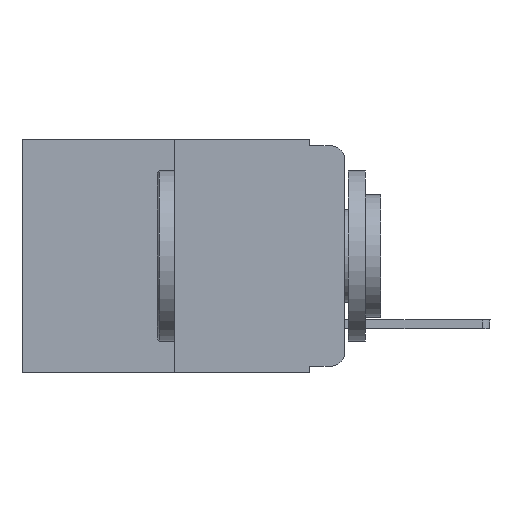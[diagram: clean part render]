
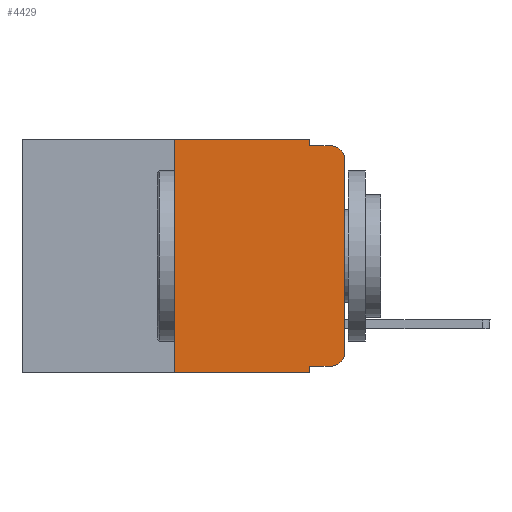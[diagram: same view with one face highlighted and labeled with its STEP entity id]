
A CAD part, left-side view. The second image highlights one B-rep face of the part: STEP entity #4429.
In plain terms, the highlighted planar face has unit normal (-1, 0, 0).
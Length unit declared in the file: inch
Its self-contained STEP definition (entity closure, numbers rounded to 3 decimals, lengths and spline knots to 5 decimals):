
#140 = VERTEX_POINT ( 'NONE', #6295 ) ;
#199 = ORIENTED_EDGE ( 'NONE', *, *, #9399, .T. ) ;
#248 = EDGE_CURVE ( 'NONE', #2056, #353, #7643, .T. ) ;
#317 = CIRCLE ( 'NONE', #6885, 0.02 ) ;
#353 = VERTEX_POINT ( 'NONE', #11382 ) ;
#426 = VECTOR ( 'NONE', #5553, 39.37008 ) ;
#587 = CARTESIAN_POINT ( 'NONE',  ( 0., 0.25, 0. ) ) ;
#712 = FACE_OUTER_BOUND ( 'NONE', #11468, .T. ) ;
#1334 = DIRECTION ( 'NONE',  ( 0., 0., -1. ) ) ;
#1338 = CARTESIAN_POINT ( 'NONE',  ( 0., 0.051, -0.01 ) ) ;
#1435 = CARTESIAN_POINT ( 'NONE',  ( 0., 0., 0. ) ) ;
#1440 = VERTEX_POINT ( 'NONE', #3270 ) ;
#1649 = CARTESIAN_POINT ( 'NONE',  ( 0., 0.02, -0.313 ) ) ;
#1845 = EDGE_CURVE ( 'NONE', #9660, #1440, #3730, .T. ) ;
#2056 = VERTEX_POINT ( 'NONE', #587 ) ;
#2116 = ORIENTED_EDGE ( 'NONE', *, *, #4659, .F. ) ;
#2437 = DIRECTION ( 'NONE',  ( 0., 0., 1. ) ) ;
#2562 = LINE ( 'NONE', #1435, #10126 ) ;
#3213 = EDGE_CURVE ( 'NONE', #9003, #10331, #8303, .T. ) ;
#3270 = CARTESIAN_POINT ( 'NONE',  ( 0., 0.02, -0.01 ) ) ;
#3324 = VECTOR ( 'NONE', #6934, 39.37008 ) ;
#3371 = DIRECTION ( 'NONE',  ( 0., -1., 0. ) ) ;
#3472 = VERTEX_POINT ( 'NONE', #9211 ) ;
#3614 = DIRECTION ( 'NONE',  ( 0., 0., -1. ) ) ;
#3730 = LINE ( 'NONE', #1338, #6246 ) ;
#3809 = CARTESIAN_POINT ( 'NONE',  ( 0., 0.02, -0.333 ) ) ;
#3892 = ORIENTED_EDGE ( 'NONE', *, *, #1845, .F. ) ;
#4140 = EDGE_CURVE ( 'NONE', #9003, #140, #12476, .T. ) ;
#4429 = ADVANCED_FACE ( 'NONE', ( #712 ), #6702, .F. ) ;
#4484 = VECTOR ( 'NONE', #7977, 39.37008 ) ;
#4570 = ORIENTED_EDGE ( 'NONE', *, *, #7966, .T. ) ;
#4659 = EDGE_CURVE ( 'NONE', #353, #9660, #10275, .T. ) ;
#4770 = DIRECTION ( 'NONE',  ( 1., 0., 0. ) ) ;
#4822 = DIRECTION ( 'NONE',  ( 0., 0., -1. ) ) ;
#5032 = VECTOR ( 'NONE', #3371, 39.37008 ) ;
#5109 = CARTESIAN_POINT ( 'NONE',  ( 0., 0.051, -0.333 ) ) ;
#5352 = VECTOR ( 'NONE', #7853, 39.37008 ) ;
#5553 = DIRECTION ( 'NONE',  ( 0., -1., 0. ) ) ;
#5767 = DIRECTION ( 'NONE',  ( 0., 0., -1. ) ) ;
#5954 = CARTESIAN_POINT ( 'NONE',  ( 0., 0.051, 0. ) ) ;
#6224 = CARTESIAN_POINT ( 'NONE',  ( 0., 0.25, -0.343 ) ) ;
#6246 = VECTOR ( 'NONE', #12232, 39.37008 ) ;
#6295 = CARTESIAN_POINT ( 'NONE',  ( 0., 0.051, -0.343 ) ) ;
#6491 = AXIS2_PLACEMENT_3D ( 'NONE', #11656, #4770, #4822 ) ;
#6660 = ORIENTED_EDGE ( 'NONE', *, *, #9619, .F. ) ;
#6702 = PLANE ( 'NONE',  #6491 ) ;
#6885 = AXIS2_PLACEMENT_3D ( 'NONE', #1649, #8663, #3614 ) ;
#6934 = DIRECTION ( 'NONE',  ( 0., 0., -1. ) ) ;
#6960 = VERTEX_POINT ( 'NONE', #6224 ) ;
#7109 = LINE ( 'NONE', #11032, #4484 ) ;
#7509 = VECTOR ( 'NONE', #1334, 39.37008 ) ;
#7643 = LINE ( 'NONE', #9274, #5032 ) ;
#7788 = CARTESIAN_POINT ( 'NONE',  ( 0., 0.051, -0.01 ) ) ;
#7853 = DIRECTION ( 'NONE',  ( 0., 0., 1. ) ) ;
#7945 = LINE ( 'NONE', #9692, #5352 ) ;
#7966 = EDGE_CURVE ( 'NONE', #10331, #10767, #317, .T. ) ;
#7977 = DIRECTION ( 'NONE',  ( 0., -1., 0. ) ) ;
#8023 = CARTESIAN_POINT ( 'NONE',  ( 0., 0.051, 0. ) ) ;
#8287 = ORIENTED_EDGE ( 'NONE', *, *, #3213, .T. ) ;
#8303 = LINE ( 'NONE', #11632, #426 ) ;
#8586 = AXIS2_PLACEMENT_3D ( 'NONE', #11627, #11546, #5767 ) ;
#8663 = DIRECTION ( 'NONE',  ( -1., 0., 0. ) ) ;
#8929 = EDGE_CURVE ( 'NONE', #6960, #140, #7109, .T. ) ;
#9003 = VERTEX_POINT ( 'NONE', #5109 ) ;
#9211 = CARTESIAN_POINT ( 'NONE',  ( 0., 0., -0.03 ) ) ;
#9274 = CARTESIAN_POINT ( 'NONE',  ( 0., 0.473, 0. ) ) ;
#9399 = EDGE_CURVE ( 'NONE', #10767, #3472, #2562, .T. ) ;
#9619 = EDGE_CURVE ( 'NONE', #6960, #2056, #7945, .T. ) ;
#9660 = VERTEX_POINT ( 'NONE', #7788 ) ;
#9692 = CARTESIAN_POINT ( 'NONE',  ( 0., 0.25, 0. ) ) ;
#10126 = VECTOR ( 'NONE', #2437, 39.37008 ) ;
#10275 = LINE ( 'NONE', #5954, #3324 ) ;
#10331 = VERTEX_POINT ( 'NONE', #3809 ) ;
#10724 = CIRCLE ( 'NONE', #8586, 0.02 ) ;
#10767 = VERTEX_POINT ( 'NONE', #11575 ) ;
#11032 = CARTESIAN_POINT ( 'NONE',  ( 0., 0.473, -0.343 ) ) ;
#11382 = CARTESIAN_POINT ( 'NONE',  ( 0., 0.051, 0. ) ) ;
#11468 = EDGE_LOOP ( 'NONE', ( #199, #12761, #3892, #2116, #12513, #6660, #11864, #12731, #8287, #4570 ) ) ;
#11546 = DIRECTION ( 'NONE',  ( -1., 0., 0. ) ) ;
#11575 = CARTESIAN_POINT ( 'NONE',  ( 0., 0., -0.313 ) ) ;
#11627 = CARTESIAN_POINT ( 'NONE',  ( 0., 0.02, -0.03 ) ) ;
#11632 = CARTESIAN_POINT ( 'NONE',  ( 0., 0.051, -0.333 ) ) ;
#11656 = CARTESIAN_POINT ( 'NONE',  ( 0., 0.473, 0. ) ) ;
#11864 = ORIENTED_EDGE ( 'NONE', *, *, #8929, .T. ) ;
#12232 = DIRECTION ( 'NONE',  ( 0., -1., 0. ) ) ;
#12476 = LINE ( 'NONE', #8023, #7509 ) ;
#12513 = ORIENTED_EDGE ( 'NONE', *, *, #248, .F. ) ;
#12731 = ORIENTED_EDGE ( 'NONE', *, *, #4140, .F. ) ;
#12761 = ORIENTED_EDGE ( 'NONE', *, *, #12793, .T. ) ;
#12793 = EDGE_CURVE ( 'NONE', #3472, #1440, #10724, .T. ) ;
